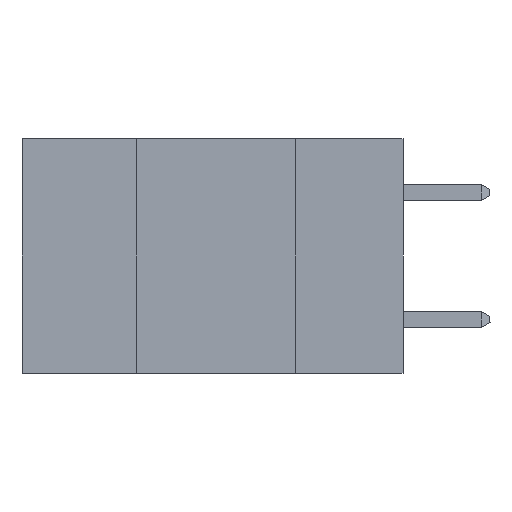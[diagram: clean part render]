
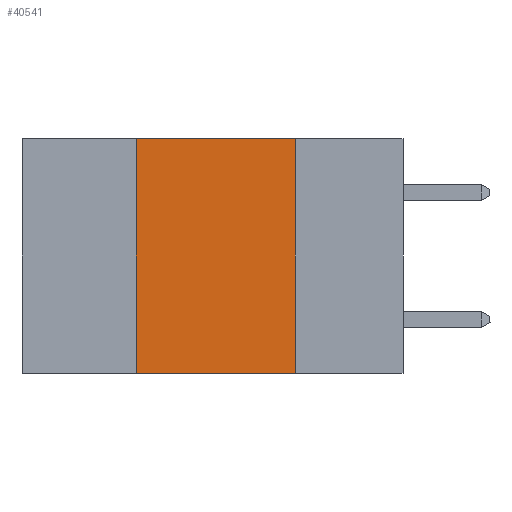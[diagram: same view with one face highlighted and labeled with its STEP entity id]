
A CAD part, left-side view. The second image highlights one B-rep face of the part: STEP entity #40541.
In plain terms, the highlighted planar face has unit normal (-1, 0, 0).
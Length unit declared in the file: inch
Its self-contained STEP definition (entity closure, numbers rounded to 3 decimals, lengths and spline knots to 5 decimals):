
#403 = FACE_OUTER_BOUND ( 'NONE', #3926, .T. ) ;
#1318 = VERTEX_POINT ( 'NONE', #38440 ) ;
#1811 = EDGE_CURVE ( 'NONE', #6456, #1318, #9664, .T. ) ;
#1954 = CARTESIAN_POINT ( 'NONE',  ( 0., 0.42, -0.37 ) ) ;
#2672 = CARTESIAN_POINT ( 'NONE',  ( 0., 0.6, 0. ) ) ;
#3087 = CARTESIAN_POINT ( 'NONE',  ( 0., 0.42, 0. ) ) ;
#3926 = EDGE_LOOP ( 'NONE', ( #40990, #25746, #15755, #30017 ) ) ;
#5642 = EDGE_CURVE ( 'NONE', #1318, #38498, #41391, .T. ) ;
#5696 = LINE ( 'NONE', #34145, #9202 ) ;
#6187 = EDGE_CURVE ( 'NONE', #6456, #37647, #7209, .T. ) ;
#6456 = VERTEX_POINT ( 'NONE', #1954 ) ;
#7209 = LINE ( 'NONE', #36365, #10205 ) ;
#8245 = VECTOR ( 'NONE', #33354, 39.37008 ) ;
#8671 = VECTOR ( 'NONE', #40988, 39.37008 ) ;
#9202 = VECTOR ( 'NONE', #37098, 39.37008 ) ;
#9664 = LINE ( 'NONE', #3087, #8671 ) ;
#10205 = VECTOR ( 'NONE', #29531, 39.37008 ) ;
#12525 = EDGE_CURVE ( 'NONE', #38498, #37647, #5696, .T. ) ;
#15755 = ORIENTED_EDGE ( 'NONE', *, *, #1811, .F. ) ;
#16100 = DIRECTION ( 'NONE',  ( 0., 0., -1. ) ) ;
#17054 = CARTESIAN_POINT ( 'NONE',  ( 0., 0.17, 0. ) ) ;
#22744 = AXIS2_PLACEMENT_3D ( 'NONE', #2672, #34347, #16100 ) ;
#25746 = ORIENTED_EDGE ( 'NONE', *, *, #5642, .F. ) ;
#25761 = CARTESIAN_POINT ( 'NONE',  ( 0., 0.6, 0. ) ) ;
#29170 = CARTESIAN_POINT ( 'NONE',  ( 0., 0.17, -0.37 ) ) ;
#29531 = DIRECTION ( 'NONE',  ( 0., -1., 0. ) ) ;
#30017 = ORIENTED_EDGE ( 'NONE', *, *, #6187, .T. ) ;
#33354 = DIRECTION ( 'NONE',  ( 0., -1., 0. ) ) ;
#34145 = CARTESIAN_POINT ( 'NONE',  ( 0., 0.17, 0. ) ) ;
#34347 = DIRECTION ( 'NONE',  ( 1., 0., 0. ) ) ;
#36365 = CARTESIAN_POINT ( 'NONE',  ( 0., 0.6, -0.37 ) ) ;
#37098 = DIRECTION ( 'NONE',  ( 0., 0., -1. ) ) ;
#37647 = VERTEX_POINT ( 'NONE', #29170 ) ;
#38440 = CARTESIAN_POINT ( 'NONE',  ( 0., 0.42, 0. ) ) ;
#38498 = VERTEX_POINT ( 'NONE', #17054 ) ;
#40541 = ADVANCED_FACE ( 'NONE', ( #403 ), #41140, .F. ) ;
#40988 = DIRECTION ( 'NONE',  ( 0., 0., 1. ) ) ;
#40990 = ORIENTED_EDGE ( 'NONE', *, *, #12525, .F. ) ;
#41140 = PLANE ( 'NONE',  #22744 ) ;
#41391 = LINE ( 'NONE', #25761, #8245 ) ;
